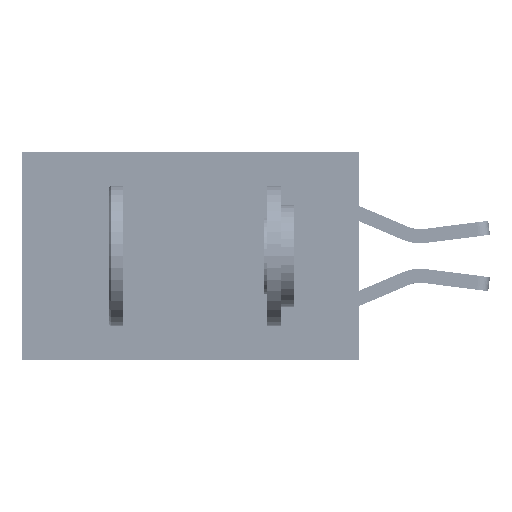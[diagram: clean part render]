
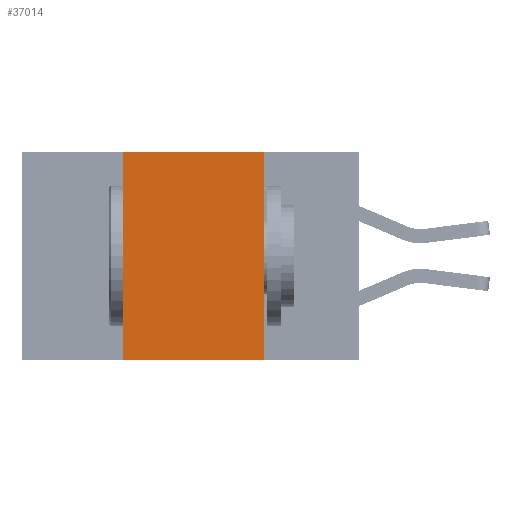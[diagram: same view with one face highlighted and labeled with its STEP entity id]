
A CAD part, left-side view. The second image highlights one B-rep face of the part: STEP entity #37014.
In plain terms, the highlighted planar face has unit normal (-1, 0, 0).
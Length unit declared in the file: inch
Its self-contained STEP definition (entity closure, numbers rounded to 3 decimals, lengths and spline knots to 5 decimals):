
#1193 = CARTESIAN_POINT ( 'NONE',  ( 0., 0.42, 0. ) ) ;
#1413 = PLANE ( 'NONE',  #48244 ) ;
#1588 = DIRECTION ( 'NONE',  ( 0., 0., -1. ) ) ;
#2567 = VECTOR ( 'NONE', #19164, 39.37008 ) ;
#3345 = EDGE_CURVE ( 'NONE', #42231, #46038, #30608, .T. ) ;
#7400 = FACE_OUTER_BOUND ( 'NONE', #10366, .T. ) ;
#10366 = EDGE_LOOP ( 'NONE', ( #16186, #48287, #28412, #46749 ) ) ;
#11347 = VERTEX_POINT ( 'NONE', #46723 ) ;
#12298 = LINE ( 'NONE', #38048, #2567 ) ;
#16186 = ORIENTED_EDGE ( 'NONE', *, *, #32125, .F. ) ;
#16225 = DIRECTION ( 'NONE',  ( 0., -1., 0. ) ) ;
#19164 = DIRECTION ( 'NONE',  ( 0., 0., -1. ) ) ;
#21502 = VECTOR ( 'NONE', #16225, 39.37008 ) ;
#21937 = LINE ( 'NONE', #33841, #29214 ) ;
#28338 = DIRECTION ( 'NONE',  ( 0., 0., 1. ) ) ;
#28412 = ORIENTED_EDGE ( 'NONE', *, *, #49804, .F. ) ;
#29214 = VECTOR ( 'NONE', #37779, 39.37008 ) ;
#29256 = EDGE_CURVE ( 'NONE', #11347, #38368, #21937, .T. ) ;
#30608 = LINE ( 'NONE', #47876, #21502 ) ;
#32125 = EDGE_CURVE ( 'NONE', #38368, #46038, #12298, .T. ) ;
#32148 = DIRECTION ( 'NONE',  ( 1., 0., 0. ) ) ;
#33024 = LINE ( 'NONE', #1193, #37952 ) ;
#33841 = CARTESIAN_POINT ( 'NONE',  ( 0., 0.6, 0. ) ) ;
#33875 = CARTESIAN_POINT ( 'NONE',  ( 0., 0.17, 0. ) ) ;
#37014 = ADVANCED_FACE ( 'NONE', ( #7400 ), #1413, .F. ) ;
#37779 = DIRECTION ( 'NONE',  ( 0., -1., 0. ) ) ;
#37952 = VECTOR ( 'NONE', #28338, 39.37008 ) ;
#38048 = CARTESIAN_POINT ( 'NONE',  ( 0., 0.17, 0. ) ) ;
#38368 = VERTEX_POINT ( 'NONE', #33875 ) ;
#42231 = VERTEX_POINT ( 'NONE', #49110 ) ;
#43918 = CARTESIAN_POINT ( 'NONE',  ( 0., 0.6, 0. ) ) ;
#46038 = VERTEX_POINT ( 'NONE', #46305 ) ;
#46305 = CARTESIAN_POINT ( 'NONE',  ( 0., 0.17, -0.37 ) ) ;
#46723 = CARTESIAN_POINT ( 'NONE',  ( 0., 0.42, 0. ) ) ;
#46749 = ORIENTED_EDGE ( 'NONE', *, *, #3345, .T. ) ;
#47876 = CARTESIAN_POINT ( 'NONE',  ( 0., 0.6, -0.37 ) ) ;
#48244 = AXIS2_PLACEMENT_3D ( 'NONE', #43918, #32148, #1588 ) ;
#48287 = ORIENTED_EDGE ( 'NONE', *, *, #29256, .F. ) ;
#49110 = CARTESIAN_POINT ( 'NONE',  ( 0., 0.42, -0.37 ) ) ;
#49804 = EDGE_CURVE ( 'NONE', #42231, #11347, #33024, .T. ) ;
